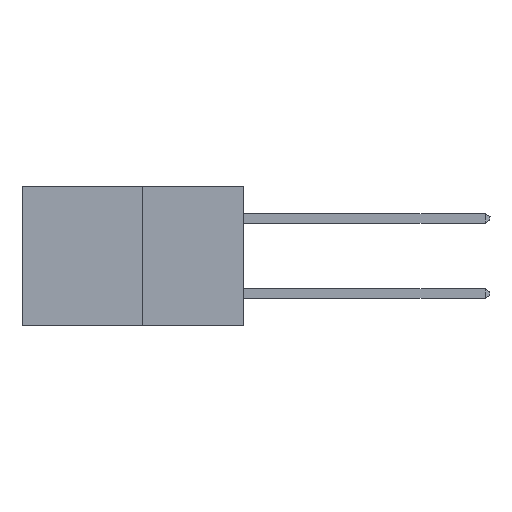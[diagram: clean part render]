
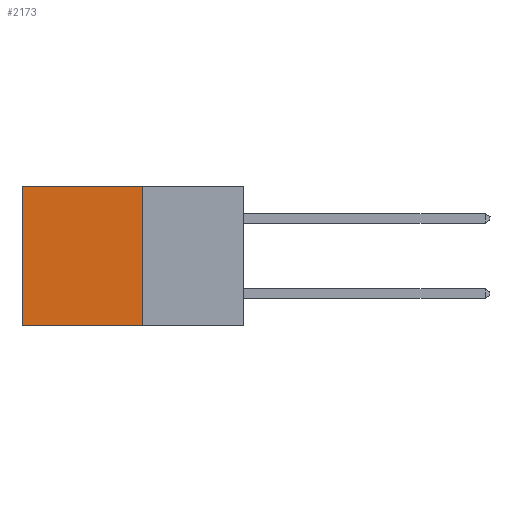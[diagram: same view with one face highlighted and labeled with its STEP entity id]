
A CAD part, left-side view. The second image highlights one B-rep face of the part: STEP entity #2173.
In plain terms, the highlighted planar face has unit normal (-1, 0, 0).
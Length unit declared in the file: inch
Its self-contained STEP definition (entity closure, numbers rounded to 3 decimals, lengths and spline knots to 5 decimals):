
#593 = ORIENTED_EDGE ( 'NONE', *, *, #1515, .F. ) ;
#610 = CARTESIAN_POINT ( 'NONE',  ( 0.277, 0.59, -0.37 ) ) ;
#812 = VECTOR ( 'NONE', #8597, 39.37008 ) ;
#890 = LINE ( 'NONE', #3930, #8592 ) ;
#1171 = VECTOR ( 'NONE', #3220, 39.37008 ) ;
#1515 = EDGE_CURVE ( 'NONE', #2520, #5404, #8514, .T. ) ;
#2173 = ADVANCED_FACE ( 'NONE', ( #7464 ), #5453, .F. ) ;
#2415 = CARTESIAN_POINT ( 'NONE',  ( 0.277, 0.59, 0. ) ) ;
#2520 = VERTEX_POINT ( 'NONE', #7344 ) ;
#2627 = ORIENTED_EDGE ( 'NONE', *, *, #8056, .T. ) ;
#3220 = DIRECTION ( 'NONE',  ( 0., 0., -1. ) ) ;
#3295 = EDGE_CURVE ( 'NONE', #5404, #6426, #890, .T. ) ;
#3466 = AXIS2_PLACEMENT_3D ( 'NONE', #7036, #5646, #3544 ) ;
#3544 = DIRECTION ( 'NONE',  ( 0., 0., -1. ) ) ;
#3930 = CARTESIAN_POINT ( 'NONE',  ( 0.277, 0.27, -0.37 ) ) ;
#3955 = EDGE_LOOP ( 'NONE', ( #4380, #6408, #593, #2627 ) ) ;
#4380 = ORIENTED_EDGE ( 'NONE', *, *, #7556, .T. ) ;
#5273 = CARTESIAN_POINT ( 'NONE',  ( 0.277, 0.27, -0.37 ) ) ;
#5400 = CARTESIAN_POINT ( 'NONE',  ( 0.277, 0.27, 0. ) ) ;
#5404 = VERTEX_POINT ( 'NONE', #5273 ) ;
#5451 = DIRECTION ( 'NONE',  ( 0., 1., 0. ) ) ;
#5453 = PLANE ( 'NONE',  #3466 ) ;
#5646 = DIRECTION ( 'NONE',  ( 1., 0., 0. ) ) ;
#6150 = DIRECTION ( 'NONE',  ( 0., 1., 0. ) ) ;
#6408 = ORIENTED_EDGE ( 'NONE', *, *, #3295, .F. ) ;
#6426 = VERTEX_POINT ( 'NONE', #610 ) ;
#6694 = VECTOR ( 'NONE', #6150, 39.37008 ) ;
#6940 = LINE ( 'NONE', #9096, #1171 ) ;
#7036 = CARTESIAN_POINT ( 'NONE',  ( 0.277, 0.27, -0.37 ) ) ;
#7344 = CARTESIAN_POINT ( 'NONE',  ( 0.277, 0.27, 0. ) ) ;
#7370 = CARTESIAN_POINT ( 'NONE',  ( 0.277, 0.27, -0.37 ) ) ;
#7464 = FACE_OUTER_BOUND ( 'NONE', #3955, .T. ) ;
#7556 = EDGE_CURVE ( 'NONE', #8079, #6426, #6940, .T. ) ;
#8056 = EDGE_CURVE ( 'NONE', #2520, #8079, #9042, .T. ) ;
#8079 = VERTEX_POINT ( 'NONE', #2415 ) ;
#8514 = LINE ( 'NONE', #7370, #812 ) ;
#8592 = VECTOR ( 'NONE', #5451, 39.37008 ) ;
#8597 = DIRECTION ( 'NONE',  ( 0., 0., -1. ) ) ;
#9042 = LINE ( 'NONE', #5400, #6694 ) ;
#9096 = CARTESIAN_POINT ( 'NONE',  ( 0.277, 0.59, -0.37 ) ) ;
